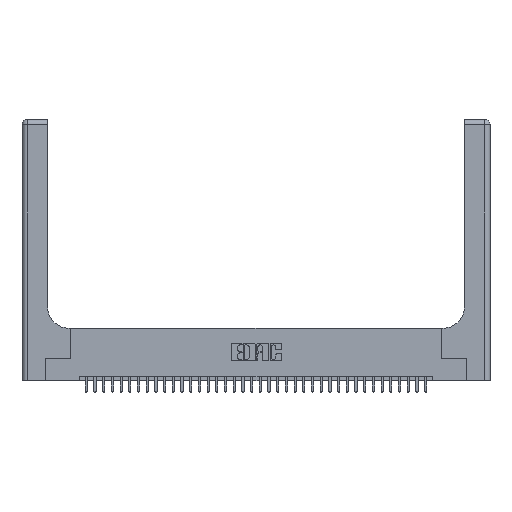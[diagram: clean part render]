
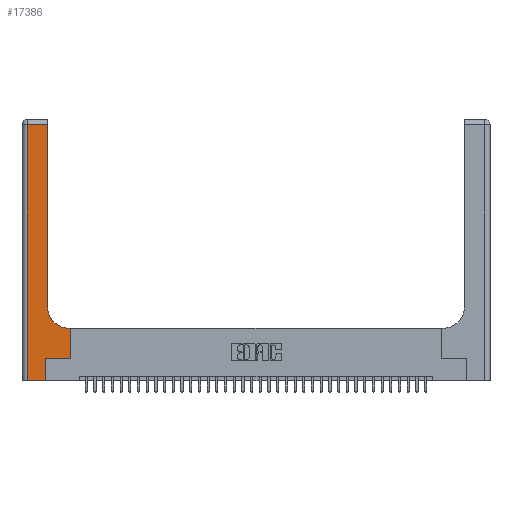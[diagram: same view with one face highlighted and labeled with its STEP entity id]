
A CAD part, top view. The second image highlights one B-rep face of the part: STEP entity #17386.
In plain terms, the highlighted planar face has unit normal (0, 0, 1).
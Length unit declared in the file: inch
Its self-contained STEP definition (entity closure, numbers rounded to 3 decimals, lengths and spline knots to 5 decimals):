
#190 = DIRECTION ( 'NONE',  ( 0., -1., 0. ) ) ;
#686 = CARTESIAN_POINT ( 'NONE',  ( 0., 2.94, 0.37 ) ) ;
#1206 = ORIENTED_EDGE ( 'NONE', *, *, #9628, .T. ) ;
#1540 = VERTEX_POINT ( 'NONE', #21902 ) ;
#1707 = DIRECTION ( 'NONE',  ( -1., 0., 0. ) ) ;
#1961 = VERTEX_POINT ( 'NONE', #6264 ) ;
#2270 = VERTEX_POINT ( 'NONE', #24858 ) ;
#2509 = EDGE_CURVE ( 'NONE', #2270, #26124, #6080, .T. ) ;
#4144 = LINE ( 'NONE', #23170, #34398 ) ;
#4592 = VERTEX_POINT ( 'NONE', #20980 ) ;
#5482 = CARTESIAN_POINT ( 'NONE',  ( 0.5585, 0.25, 0.37 ) ) ;
#5984 = CARTESIAN_POINT ( 'NONE',  ( 0.5415, 0.85, 0.37 ) ) ;
#6080 = LINE ( 'NONE', #14474, #20286 ) ;
#6161 = DIRECTION ( 'NONE',  ( 0., 1., 0. ) ) ;
#6257 = EDGE_CURVE ( 'NONE', #23468, #33331, #23415, .T. ) ;
#6264 = CARTESIAN_POINT ( 'NONE',  ( 0.2915, 2.94, 0.37 ) ) ;
#6343 = LINE ( 'NONE', #5482, #21441 ) ;
#6576 = CARTESIAN_POINT ( 'NONE',  ( 0., 3., 0.37 ) ) ;
#6846 = LINE ( 'NONE', #30633, #28609 ) ;
#8648 = EDGE_CURVE ( 'NONE', #4592, #24364, #6846, .T. ) ;
#8853 = DIRECTION ( 'NONE',  ( 1., 0., 0. ) ) ;
#8873 = EDGE_LOOP ( 'NONE', ( #14026, #1206, #14073, #13285, #9541, #28925, #33518, #11907, #23637 ) ) ;
#9402 = EDGE_CURVE ( 'NONE', #24364, #23468, #6343, .T. ) ;
#9541 = ORIENTED_EDGE ( 'NONE', *, *, #27001, .T. ) ;
#9624 = CARTESIAN_POINT ( 'NONE',  ( 0.5585, 0.6, 0.37 ) ) ;
#9628 = EDGE_CURVE ( 'NONE', #1961, #2270, #36107, .T. ) ;
#10425 = CARTESIAN_POINT ( 'NONE',  ( 0.5585, 0.25, 0.37 ) ) ;
#10778 = DIRECTION ( 'NONE',  ( 1., 0., 0. ) ) ;
#11907 = ORIENTED_EDGE ( 'NONE', *, *, #6257, .T. ) ;
#12553 = VECTOR ( 'NONE', #32551, 39.37008 ) ;
#13285 = ORIENTED_EDGE ( 'NONE', *, *, #23562, .T. ) ;
#13800 = VECTOR ( 'NONE', #33677, 39.37008 ) ;
#14026 = ORIENTED_EDGE ( 'NONE', *, *, #23836, .T. ) ;
#14073 = ORIENTED_EDGE ( 'NONE', *, *, #2509, .T. ) ;
#14268 = LINE ( 'NONE', #18554, #28448 ) ;
#14474 = CARTESIAN_POINT ( 'NONE',  ( 0.06, 3., 0.37 ) ) ;
#15886 = VECTOR ( 'NONE', #1707, 39.37008 ) ;
#16481 = LINE ( 'NONE', #33560, #13800 ) ;
#16952 = DIRECTION ( 'NONE',  ( 0., 1., 0. ) ) ;
#17386 = ADVANCED_FACE ( 'NONE', ( #29136 ), #18038, .F. ) ;
#18038 = PLANE ( 'NONE',  #34367 ) ;
#18554 = CARTESIAN_POINT ( 'NONE',  ( 0., 0., 0.37 ) ) ;
#19265 = CARTESIAN_POINT ( 'NONE',  ( 0.06, 0., 0.37 ) ) ;
#20197 = CARTESIAN_POINT ( 'NONE',  ( 0.269, 0., 0.37 ) ) ;
#20286 = VECTOR ( 'NONE', #190, 39.37008 ) ;
#20980 = CARTESIAN_POINT ( 'NONE',  ( 0.269, 0.25, 0.37 ) ) ;
#21009 = CIRCLE ( 'NONE', #25385, 0.25 ) ;
#21033 = EDGE_CURVE ( 'NONE', #33331, #1540, #21009, .T. ) ;
#21441 = VECTOR ( 'NONE', #16952, 39.37008 ) ;
#21902 = CARTESIAN_POINT ( 'NONE',  ( 0.2915, 0.85, 0.37 ) ) ;
#23170 = CARTESIAN_POINT ( 'NONE',  ( 0.269, 0., 0.37 ) ) ;
#23415 = LINE ( 'NONE', #35675, #15886 ) ;
#23468 = VERTEX_POINT ( 'NONE', #9624 ) ;
#23562 = EDGE_CURVE ( 'NONE', #26124, #24626, #14268, .T. ) ;
#23637 = ORIENTED_EDGE ( 'NONE', *, *, #21033, .T. ) ;
#23703 = DIRECTION ( 'NONE',  ( -1., 0., 0. ) ) ;
#23836 = EDGE_CURVE ( 'NONE', #1540, #1961, #16481, .T. ) ;
#24233 = DIRECTION ( 'NONE',  ( 1., 0., 0. ) ) ;
#24364 = VERTEX_POINT ( 'NONE', #10425 ) ;
#24626 = VERTEX_POINT ( 'NONE', #20197 ) ;
#24858 = CARTESIAN_POINT ( 'NONE',  ( 0.06, 2.94, 0.37 ) ) ;
#25385 = AXIS2_PLACEMENT_3D ( 'NONE', #5984, #25843, #8853 ) ;
#25843 = DIRECTION ( 'NONE',  ( 0., 0., -1. ) ) ;
#26124 = VERTEX_POINT ( 'NONE', #19265 ) ;
#27001 = EDGE_CURVE ( 'NONE', #24626, #4592, #4144, .T. ) ;
#28318 = CARTESIAN_POINT ( 'NONE',  ( 0.5415, 0.6, 0.37 ) ) ;
#28448 = VECTOR ( 'NONE', #24233, 39.37008 ) ;
#28609 = VECTOR ( 'NONE', #10778, 39.37008 ) ;
#28925 = ORIENTED_EDGE ( 'NONE', *, *, #8648, .T. ) ;
#29136 = FACE_OUTER_BOUND ( 'NONE', #8873, .T. ) ;
#30633 = CARTESIAN_POINT ( 'NONE',  ( 0.269, 0.25, 0.37 ) ) ;
#32551 = DIRECTION ( 'NONE',  ( -1., 0., 0. ) ) ;
#33331 = VERTEX_POINT ( 'NONE', #28318 ) ;
#33518 = ORIENTED_EDGE ( 'NONE', *, *, #9402, .T. ) ;
#33560 = CARTESIAN_POINT ( 'NONE',  ( 0.2915, 3., 0.37 ) ) ;
#33677 = DIRECTION ( 'NONE',  ( 0., 1., 0. ) ) ;
#34367 = AXIS2_PLACEMENT_3D ( 'NONE', #6576, #34895, #23703 ) ;
#34398 = VECTOR ( 'NONE', #6161, 39.37008 ) ;
#34895 = DIRECTION ( 'NONE',  ( 0., 0., -1. ) ) ;
#35675 = CARTESIAN_POINT ( 'NONE',  ( 0.2915, 0.6, 0.37 ) ) ;
#36107 = LINE ( 'NONE', #686, #12553 ) ;
